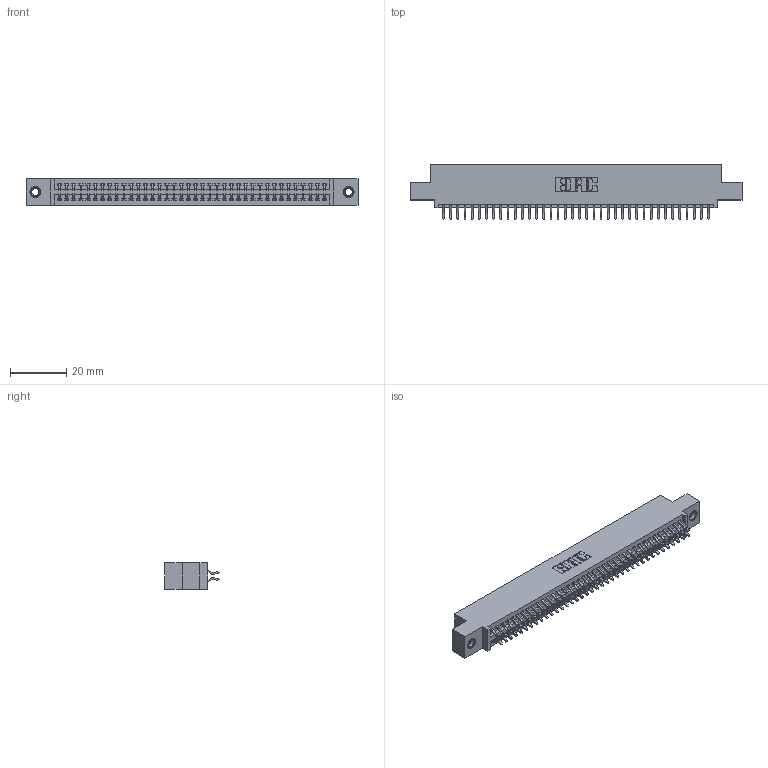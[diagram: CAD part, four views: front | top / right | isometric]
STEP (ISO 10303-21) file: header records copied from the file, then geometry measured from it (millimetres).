
FILE_DESCRIPTION (( 'STEP AP203' ), '1' );
FILE_NAME ('395-076-556-507.STEP', '2018-11-27T22:26:28', ( '' ), ( '' ), 'SwSTEP 2.0', 'SolidWorks 2016', '' );
FILE_SCHEMA (( 'CONFIG_CONTROL_DESIGN' ));
Length unit declared in the file: inch
Products named in the file (4): 345-292-001_556 Tail; 345 Part_0.110 Offset - 0.156 Dia-TI; 395-076-556-507; 345-250-001_345-250-005-103
Assembly tree (79 placements, depth 2):
  395-076-556-507
    345 Part_0.110 Offset - 0.156 Dia-TI
    345-292-001_556 Tail  x76
    345-250-001_345-250-005-103  x2
Bounding box: 117.73 x 19.24 x 9.4 mm (x, y, z)
Volume: 11309.3 mm3; surface area: 16693.8 mm2
Topology: 79 solids, 79 shells, 4446 faces, 13181 edges, 8678 vertices
Faces by surface type: plane 2928, cylinder 1502, cone 12, torus 4
Entity records: 31892 total; most frequent: CARTESIAN_POINT 5347, ORIENTED_EDGE 5262, DIRECTION 4733, EDGE_CURVE 2631, LINE 2319, VECTOR 2319, VERTEX_POINT 1748, AXIS2_PLACEMENT_3D 1207
